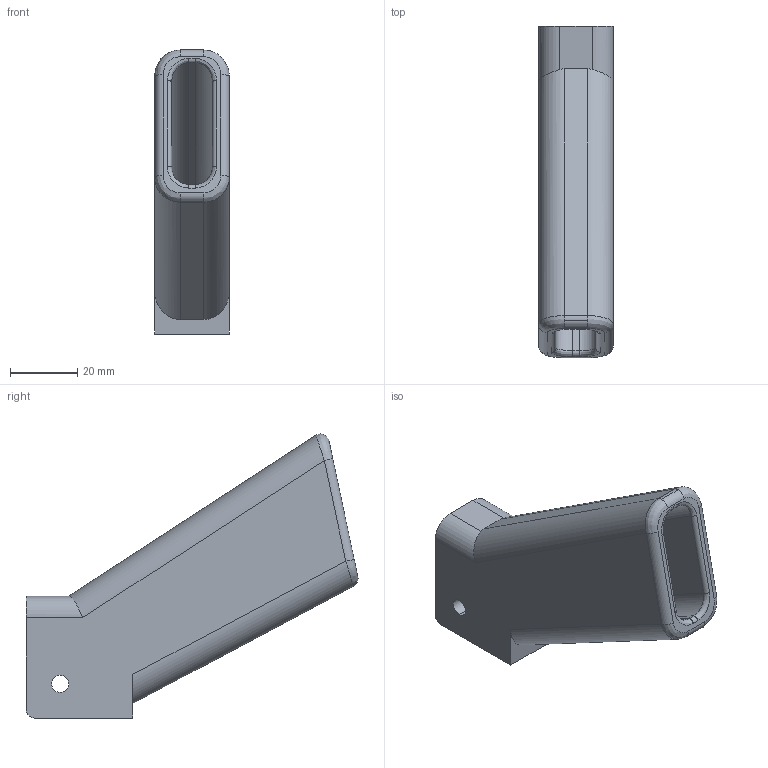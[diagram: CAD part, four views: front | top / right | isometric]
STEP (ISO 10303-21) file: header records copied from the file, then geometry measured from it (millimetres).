
FILE_DESCRIPTION (( 'STEP AP214' ), '1' );
FILE_NAME ('GripRemodeled.STEP', '2013-05-27T22:43:48', ( 'Asher' ), ( '' ), 'SwSTEP 2.0', 'SolidWorks 2013', '' );
FILE_SCHEMA (( 'AUTOMOTIVE_DESIGN' ));
Length unit declared in the file: millimetre
Products named in the file (1): GripRemodeled
Bounding box: 22.23 x 98.69 x 84.44 mm (x, y, z)
Volume: 57730.2 mm3; surface area: 20625.1 mm2
Topology: 1 solids, 1 shells, 52 faces, 131 edges, 82 vertices
Faces by surface type: cylinder 25, plane 19, bspline 8
Entity records: 1847 total; most frequent: CARTESIAN_POINT 640, ORIENTED_EDGE 262, DIRECTION 227, EDGE_CURVE 131, VERTEX_POINT 82, AXIS2_PLACEMENT_3D 77, VECTOR 73, LINE 73
